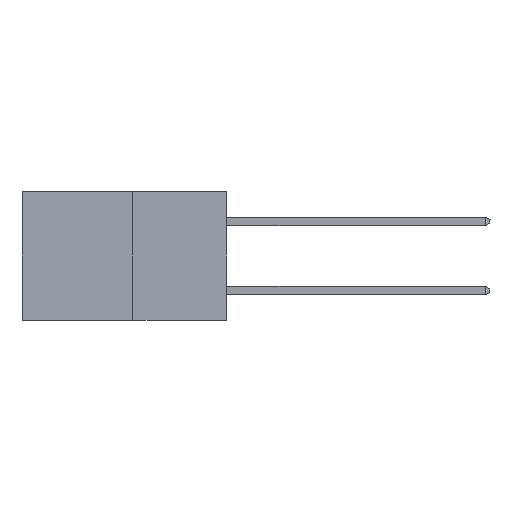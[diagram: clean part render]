
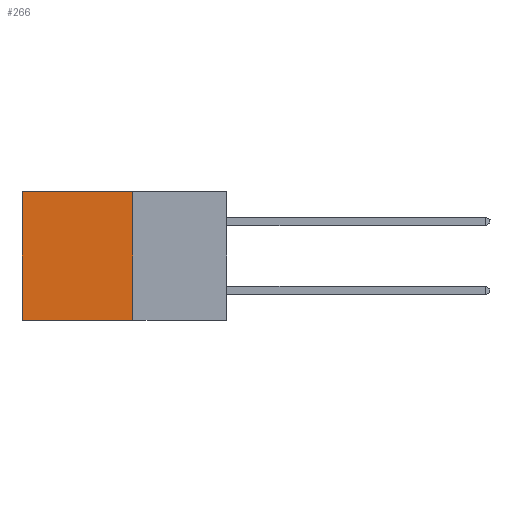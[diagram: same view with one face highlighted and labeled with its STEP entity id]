
A CAD part, left-side view. The second image highlights one B-rep face of the part: STEP entity #266.
In plain terms, the highlighted planar face has unit normal (-1, 0, 0).
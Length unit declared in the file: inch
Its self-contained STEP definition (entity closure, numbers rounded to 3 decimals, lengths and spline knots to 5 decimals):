
#266 = ADVANCED_FACE ( 'NONE', ( #5457 ), #6562, .F. ) ;
#595 = VECTOR ( 'NONE', #7808, 39.37008 ) ;
#717 = LINE ( 'NONE', #4817, #5967 ) ;
#1224 = CARTESIAN_POINT ( 'NONE',  ( 0.277, 0.27, -0.37 ) ) ;
#1567 = CARTESIAN_POINT ( 'NONE',  ( 0.277, 0.27, -0.37 ) ) ;
#1808 = VERTEX_POINT ( 'NONE', #3648 ) ;
#2010 = CARTESIAN_POINT ( 'NONE',  ( 0.277, 0.59, -0.37 ) ) ;
#2378 = EDGE_CURVE ( 'NONE', #1808, #3570, #8280, .T. ) ;
#2484 = LINE ( 'NONE', #4358, #595 ) ;
#2601 = DIRECTION ( 'NONE',  ( 0., 0., -1. ) ) ;
#2780 = EDGE_CURVE ( 'NONE', #1808, #7775, #2484, .T. ) ;
#3009 = EDGE_CURVE ( 'NONE', #7775, #4318, #717, .T. ) ;
#3110 = DIRECTION ( 'NONE',  ( 1., 0., 0. ) ) ;
#3171 = ORIENTED_EDGE ( 'NONE', *, *, #4104, .F. ) ;
#3197 = DIRECTION ( 'NONE',  ( 0., 0., -1. ) ) ;
#3570 = VERTEX_POINT ( 'NONE', #1567 ) ;
#3648 = CARTESIAN_POINT ( 'NONE',  ( 0.277, 0.27, 0. ) ) ;
#3822 = DIRECTION ( 'NONE',  ( 0., 0., -1. ) ) ;
#4104 = EDGE_CURVE ( 'NONE', #3570, #4318, #4859, .T. ) ;
#4318 = VERTEX_POINT ( 'NONE', #2010 ) ;
#4358 = CARTESIAN_POINT ( 'NONE',  ( 0.277, 0.27, 0. ) ) ;
#4817 = CARTESIAN_POINT ( 'NONE',  ( 0.277, 0.59, -0.37 ) ) ;
#4859 = LINE ( 'NONE', #8074, #8170 ) ;
#4927 = ORIENTED_EDGE ( 'NONE', *, *, #2378, .F. ) ;
#5302 = EDGE_LOOP ( 'NONE', ( #8234, #3171, #4927, #8411 ) ) ;
#5457 = FACE_OUTER_BOUND ( 'NONE', #5302, .T. ) ;
#5967 = VECTOR ( 'NONE', #2601, 39.37008 ) ;
#6562 = PLANE ( 'NONE',  #7894 ) ;
#6605 = VECTOR ( 'NONE', #3197, 39.37008 ) ;
#7007 = CARTESIAN_POINT ( 'NONE',  ( 0.277, 0.27, -0.37 ) ) ;
#7775 = VERTEX_POINT ( 'NONE', #8382 ) ;
#7808 = DIRECTION ( 'NONE',  ( 0., 1., 0. ) ) ;
#7894 = AXIS2_PLACEMENT_3D ( 'NONE', #1224, #3110, #3822 ) ;
#8030 = DIRECTION ( 'NONE',  ( 0., 1., 0. ) ) ;
#8074 = CARTESIAN_POINT ( 'NONE',  ( 0.277, 0.27, -0.37 ) ) ;
#8170 = VECTOR ( 'NONE', #8030, 39.37008 ) ;
#8234 = ORIENTED_EDGE ( 'NONE', *, *, #3009, .T. ) ;
#8280 = LINE ( 'NONE', #7007, #6605 ) ;
#8382 = CARTESIAN_POINT ( 'NONE',  ( 0.277, 0.59, 0. ) ) ;
#8411 = ORIENTED_EDGE ( 'NONE', *, *, #2780, .T. ) ;
